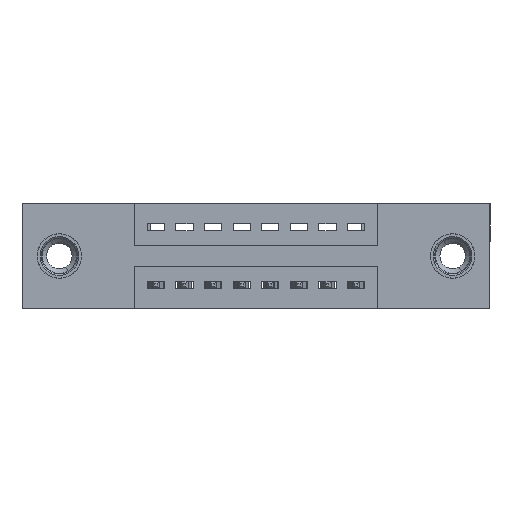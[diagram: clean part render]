
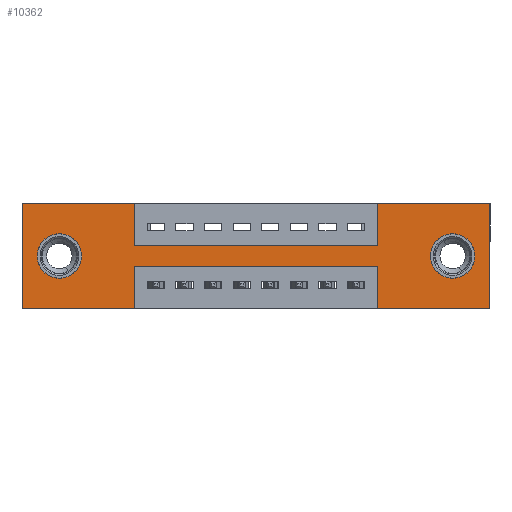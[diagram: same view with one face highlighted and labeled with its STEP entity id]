
A CAD part, front view. The second image highlights one B-rep face of the part: STEP entity #10362.
In plain terms, the highlighted planar face has unit normal (0, -1, 0).
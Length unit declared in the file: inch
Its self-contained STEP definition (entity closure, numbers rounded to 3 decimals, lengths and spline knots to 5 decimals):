
#69 = CARTESIAN_POINT ( 'NONE',  ( 1.2425, 0., -0.37 ) ) ;
#225 = VERTEX_POINT ( 'NONE', #10671 ) ;
#377 = EDGE_CURVE ( 'NONE', #10552, #379, #4509, .T. ) ;
#379 = VERTEX_POINT ( 'NONE', #5843 ) ;
#396 = LINE ( 'NONE', #11176, #10843 ) ;
#407 = ORIENTED_EDGE ( 'NONE', *, *, #377, .F. ) ;
#428 = LINE ( 'NONE', #1010, #3635 ) ;
#571 = LINE ( 'NONE', #12028, #6833 ) ;
#864 = VERTEX_POINT ( 'NONE', #8117 ) ;
#916 = DIRECTION ( 'NONE',  ( 0., 1., 0. ) ) ;
#987 = VERTEX_POINT ( 'NONE', #1422 ) ;
#1005 = ORIENTED_EDGE ( 'NONE', *, *, #10083, .T. ) ;
#1010 = CARTESIAN_POINT ( 'NONE',  ( 0., 0., -0.37 ) ) ;
#1021 = VERTEX_POINT ( 'NONE', #7286 ) ;
#1085 = DIRECTION ( 'NONE',  ( 0., 0., 1. ) ) ;
#1336 = AXIS2_PLACEMENT_3D ( 'NONE', #2836, #916, #1888 ) ;
#1340 = ORIENTED_EDGE ( 'NONE', *, *, #11290, .F. ) ;
#1386 = CARTESIAN_POINT ( 'NONE',  ( 0.13, 0., -0.107 ) ) ;
#1422 = CARTESIAN_POINT ( 'NONE',  ( 0.3925, 0., -0.15 ) ) ;
#1461 = LINE ( 'NONE', #4416, #4830 ) ;
#1465 = DIRECTION ( 'NONE',  ( 0., 0., -1. ) ) ;
#1885 = LINE ( 'NONE', #6613, #2199 ) ;
#1888 = DIRECTION ( 'NONE',  ( 0., 0., -1. ) ) ;
#2199 = VECTOR ( 'NONE', #3603, 39.37008 ) ;
#2344 = CARTESIAN_POINT ( 'NONE',  ( 0., 0., -0.37 ) ) ;
#2420 = CARTESIAN_POINT ( 'NONE',  ( 0.3925, 0., -0.22 ) ) ;
#2463 = CARTESIAN_POINT ( 'NONE',  ( 0.3925, 0., 0. ) ) ;
#2676 = VECTOR ( 'NONE', #1465, 39.37008 ) ;
#2836 = CARTESIAN_POINT ( 'NONE',  ( 1.505, 0., -0.185 ) ) ;
#2910 = CARTESIAN_POINT ( 'NONE',  ( 1.635, 0., -0.37 ) ) ;
#2982 = DIRECTION ( 'NONE',  ( -1., 0., 0. ) ) ;
#3016 = VERTEX_POINT ( 'NONE', #9688 ) ;
#3023 = VECTOR ( 'NONE', #1085, 39.37008 ) ;
#3603 = DIRECTION ( 'NONE',  ( 0., 0., -1. ) ) ;
#3620 = EDGE_CURVE ( 'NONE', #225, #7929, #5204, .T. ) ;
#3635 = VECTOR ( 'NONE', #2982, 39.37008 ) ;
#3831 = VERTEX_POINT ( 'NONE', #1386 ) ;
#3895 = VECTOR ( 'NONE', #7864, 39.37008 ) ;
#3928 = LINE ( 'NONE', #10895, #3023 ) ;
#3947 = CARTESIAN_POINT ( 'NONE',  ( 0.3925, 0., -0.37 ) ) ;
#4003 = EDGE_CURVE ( 'NONE', #864, #3831, #10256, .T. ) ;
#4075 = VERTEX_POINT ( 'NONE', #9829 ) ;
#4080 = ORIENTED_EDGE ( 'NONE', *, *, #12345, .F. ) ;
#4416 = CARTESIAN_POINT ( 'NONE',  ( 0., 0., 0. ) ) ;
#4443 = ORIENTED_EDGE ( 'NONE', *, *, #10470, .F. ) ;
#4496 = CARTESIAN_POINT ( 'NONE',  ( 0.3925, 0., -0.15 ) ) ;
#4509 = LINE ( 'NONE', #3947, #3895 ) ;
#4553 = DIRECTION ( 'NONE',  ( 0., 0., 1. ) ) ;
#4830 = VECTOR ( 'NONE', #8411, 39.37008 ) ;
#5026 = EDGE_CURVE ( 'NONE', #4075, #7123, #10062, .T. ) ;
#5088 = CARTESIAN_POINT ( 'NONE',  ( 1.505, 0., -0.107 ) ) ;
#5204 = CIRCLE ( 'NONE', #12394, 0.078 ) ;
#5489 = ORIENTED_EDGE ( 'NONE', *, *, #9771, .F. ) ;
#5549 = CARTESIAN_POINT ( 'NONE',  ( 0.13, 0., -0.185 ) ) ;
#5691 = ORIENTED_EDGE ( 'NONE', *, *, #5026, .F. ) ;
#5733 = EDGE_CURVE ( 'NONE', #1021, #6072, #1885, .T. ) ;
#5843 = CARTESIAN_POINT ( 'NONE',  ( 0.3925, 0., -0.37 ) ) ;
#5860 = CARTESIAN_POINT ( 'NONE',  ( 1.505, 0., -0.185 ) ) ;
#6067 = FACE_BOUND ( 'NONE', #12605, .T. ) ;
#6072 = VERTEX_POINT ( 'NONE', #2910 ) ;
#6132 = CARTESIAN_POINT ( 'NONE',  ( 0., 0., -0.37 ) ) ;
#6250 = AXIS2_PLACEMENT_3D ( 'NONE', #2344, #11149, #11016 ) ;
#6259 = EDGE_LOOP ( 'NONE', ( #9225, #7423 ) ) ;
#6496 = DIRECTION ( 'NONE',  ( 0., 0., 1. ) ) ;
#6613 = CARTESIAN_POINT ( 'NONE',  ( 1.635, 0., 0. ) ) ;
#6833 = VECTOR ( 'NONE', #8376, 39.37008 ) ;
#6965 = VECTOR ( 'NONE', #11649, 39.37008 ) ;
#6974 = FACE_BOUND ( 'NONE', #6259, .T. ) ;
#7123 = VERTEX_POINT ( 'NONE', #9730 ) ;
#7286 = CARTESIAN_POINT ( 'NONE',  ( 1.635, 0., 0. ) ) ;
#7371 = ORIENTED_EDGE ( 'NONE', *, *, #11112, .F. ) ;
#7423 = ORIENTED_EDGE ( 'NONE', *, *, #3620, .T. ) ;
#7438 = VERTEX_POINT ( 'NONE', #10762 ) ;
#7706 = ORIENTED_EDGE ( 'NONE', *, *, #10568, .F. ) ;
#7806 = AXIS2_PLACEMENT_3D ( 'NONE', #9459, #10454, #4553 ) ;
#7864 = DIRECTION ( 'NONE',  ( 0., 0., -1. ) ) ;
#7929 = VERTEX_POINT ( 'NONE', #5088 ) ;
#8021 = EDGE_CURVE ( 'NONE', #379, #7438, #12045, .T. ) ;
#8043 = PLANE ( 'NONE',  #6250 ) ;
#8061 = VECTOR ( 'NONE', #12483, 39.37008 ) ;
#8117 = CARTESIAN_POINT ( 'NONE',  ( 0.13, 0., -0.263 ) ) ;
#8354 = LINE ( 'NONE', #2463, #2676 ) ;
#8365 = FACE_OUTER_BOUND ( 'NONE', #8491, .T. ) ;
#8376 = DIRECTION ( 'NONE',  ( 0., 0., 1. ) ) ;
#8411 = DIRECTION ( 'NONE',  ( 1., 0., 0. ) ) ;
#8491 = EDGE_LOOP ( 'NONE', ( #407, #7371, #12743, #1340, #9529, #4443, #5691, #11052, #7706, #4080, #5489, #12039 ) ) ;
#8511 = LINE ( 'NONE', #4496, #8061 ) ;
#8531 = ORIENTED_EDGE ( 'NONE', *, *, #4003, .T. ) ;
#8635 = VECTOR ( 'NONE', #10506, 39.37008 ) ;
#8733 = EDGE_CURVE ( 'NONE', #7929, #225, #9636, .T. ) ;
#8946 = DIRECTION ( 'NONE',  ( 0., 1., 0. ) ) ;
#9082 = DIRECTION ( 'NONE',  ( 1., 0., 0. ) ) ;
#9225 = ORIENTED_EDGE ( 'NONE', *, *, #8733, .T. ) ;
#9230 = DIRECTION ( 'NONE',  ( -1., 0., 0. ) ) ;
#9362 = VECTOR ( 'NONE', #9230, 39.37008 ) ;
#9399 = DIRECTION ( 'NONE',  ( 0., 0., -1. ) ) ;
#9459 = CARTESIAN_POINT ( 'NONE',  ( 0.13, 0., -0.185 ) ) ;
#9529 = ORIENTED_EDGE ( 'NONE', *, *, #5733, .F. ) ;
#9538 = CARTESIAN_POINT ( 'NONE',  ( 0.3925, 0., -0.22 ) ) ;
#9594 = CARTESIAN_POINT ( 'NONE',  ( 1.2425, 0., 0. ) ) ;
#9636 = CIRCLE ( 'NONE', #1336, 0.078 ) ;
#9688 = CARTESIAN_POINT ( 'NONE',  ( 0., 0., 0. ) ) ;
#9730 = CARTESIAN_POINT ( 'NONE',  ( 1.2425, 0., 0. ) ) ;
#9756 = VERTEX_POINT ( 'NONE', #10996 ) ;
#9771 = EDGE_CURVE ( 'NONE', #7438, #3016, #571, .T. ) ;
#9829 = CARTESIAN_POINT ( 'NONE',  ( 1.2425, 0., -0.15 ) ) ;
#10062 = LINE ( 'NONE', #9594, #6965 ) ;
#10083 = EDGE_CURVE ( 'NONE', #3831, #864, #11825, .T. ) ;
#10256 = CIRCLE ( 'NONE', #7806, 0.078 ) ;
#10362 = ADVANCED_FACE ( 'NONE', ( #6974, #6067, #8365 ), #8043, .T. ) ;
#10454 = DIRECTION ( 'NONE',  ( 0., 1., 0. ) ) ;
#10470 = EDGE_CURVE ( 'NONE', #7123, #1021, #396, .T. ) ;
#10506 = DIRECTION ( 'NONE',  ( -1., 0., 0. ) ) ;
#10552 = VERTEX_POINT ( 'NONE', #2420 ) ;
#10568 = EDGE_CURVE ( 'NONE', #9756, #987, #8354, .T. ) ;
#10671 = CARTESIAN_POINT ( 'NONE',  ( 1.505, 0., -0.263 ) ) ;
#10762 = CARTESIAN_POINT ( 'NONE',  ( 0., 0., -0.37 ) ) ;
#10843 = VECTOR ( 'NONE', #9082, 39.37008 ) ;
#10895 = CARTESIAN_POINT ( 'NONE',  ( 1.2425, 0., -0.37 ) ) ;
#10996 = CARTESIAN_POINT ( 'NONE',  ( 0.3925, 0., 0. ) ) ;
#11016 = DIRECTION ( 'NONE',  ( 0., 0., -1. ) ) ;
#11052 = ORIENTED_EDGE ( 'NONE', *, *, #12298, .F. ) ;
#11112 = EDGE_CURVE ( 'NONE', #11183, #10552, #11627, .T. ) ;
#11149 = DIRECTION ( 'NONE',  ( 0., -1., 0. ) ) ;
#11176 = CARTESIAN_POINT ( 'NONE',  ( 0., 0., 0. ) ) ;
#11183 = VERTEX_POINT ( 'NONE', #12543 ) ;
#11290 = EDGE_CURVE ( 'NONE', #6072, #12244, #428, .T. ) ;
#11627 = LINE ( 'NONE', #9538, #8635 ) ;
#11649 = DIRECTION ( 'NONE',  ( 0., 0., 1. ) ) ;
#11655 = EDGE_CURVE ( 'NONE', #12244, #11183, #3928, .T. ) ;
#11825 = CIRCLE ( 'NONE', #12427, 0.078 ) ;
#12028 = CARTESIAN_POINT ( 'NONE',  ( 0., 0., 0. ) ) ;
#12039 = ORIENTED_EDGE ( 'NONE', *, *, #8021, .F. ) ;
#12045 = LINE ( 'NONE', #6132, #9362 ) ;
#12244 = VERTEX_POINT ( 'NONE', #69 ) ;
#12298 = EDGE_CURVE ( 'NONE', #987, #4075, #8511, .T. ) ;
#12345 = EDGE_CURVE ( 'NONE', #3016, #9756, #1461, .T. ) ;
#12394 = AXIS2_PLACEMENT_3D ( 'NONE', #5860, #8946, #9399 ) ;
#12427 = AXIS2_PLACEMENT_3D ( 'NONE', #5549, #12450, #6496 ) ;
#12450 = DIRECTION ( 'NONE',  ( 0., 1., 0. ) ) ;
#12483 = DIRECTION ( 'NONE',  ( 1., 0., 0. ) ) ;
#12543 = CARTESIAN_POINT ( 'NONE',  ( 1.2425, 0., -0.22 ) ) ;
#12605 = EDGE_LOOP ( 'NONE', ( #1005, #8531 ) ) ;
#12743 = ORIENTED_EDGE ( 'NONE', *, *, #11655, .F. ) ;
